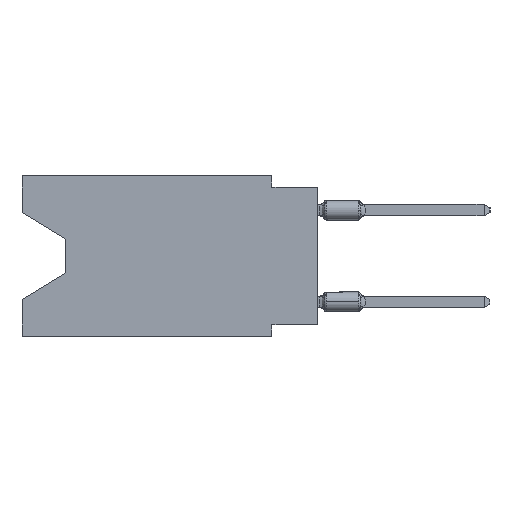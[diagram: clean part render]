
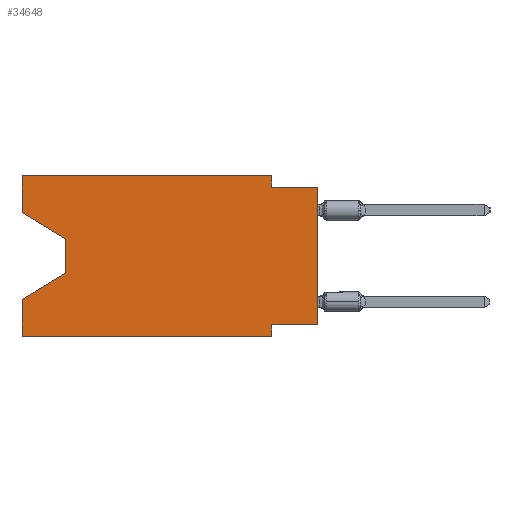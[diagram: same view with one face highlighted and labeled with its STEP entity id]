
A CAD part, left-side view. The second image highlights one B-rep face of the part: STEP entity #34648.
In plain terms, the highlighted planar face has unit normal (-1, 0, 0).
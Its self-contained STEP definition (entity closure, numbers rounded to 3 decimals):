
#612 = CARTESIAN_POINT ( 'NONE',  ( 0., 16.383, -2.038 ) ) ;
#839 = VECTOR ( 'NONE', #7871, 1000. ) ;
#1171 = EDGE_CURVE ( 'NONE', #26088, #17224, #35186, .T. ) ;
#1214 = VERTEX_POINT ( 'NONE', #32390 ) ;
#1535 = EDGE_CURVE ( 'NONE', #28753, #13794, #11944, .T. ) ;
#1687 = EDGE_CURVE ( 'NONE', #27810, #31201, #30446, .T. ) ;
#2777 = LINE ( 'NONE', #36775, #5732 ) ;
#3425 = CARTESIAN_POINT ( 'NONE',  ( 0., 16.383, 0. ) ) ;
#3776 = DIRECTION ( 'NONE',  ( 0., 0., 1. ) ) ;
#4804 = ORIENTED_EDGE ( 'NONE', *, *, #29237, .F. ) ;
#5156 = VECTOR ( 'NONE', #9319, 1000. ) ;
#5525 = EDGE_CURVE ( 'NONE', #13794, #11250, #17194, .T. ) ;
#5732 = VECTOR ( 'NONE', #28670, 1000. ) ;
#6398 = DIRECTION ( 'NONE',  ( 0., -1., 0. ) ) ;
#6976 = VECTOR ( 'NONE', #7171, 1000. ) ;
#7171 = DIRECTION ( 'NONE',  ( 0., -1., 0. ) ) ;
#7252 = ORIENTED_EDGE ( 'NONE', *, *, #5525, .F. ) ;
#7714 = CARTESIAN_POINT ( 'NONE',  ( 0., 16.383, -6.852 ) ) ;
#7871 = DIRECTION ( 'NONE',  ( 0., 0., -1. ) ) ;
#8777 = EDGE_LOOP ( 'NONE', ( #12455, #16822, #10745, #16127, #31395, #31685, #4804, #11117, #10557, #10235, #7252, #36905 ) ) ;
#9194 = PLANE ( 'NONE',  #30780 ) ;
#9319 = DIRECTION ( 'NONE',  ( 0., -1., 0. ) ) ;
#9607 = EDGE_CURVE ( 'NONE', #31598, #17224, #24558, .T. ) ;
#9770 = CARTESIAN_POINT ( 'NONE',  ( 0., 13.97, -3.505 ) ) ;
#10235 = ORIENTED_EDGE ( 'NONE', *, *, #22804, .F. ) ;
#10408 = CARTESIAN_POINT ( 'NONE',  ( 0., 16.383, -8.89 ) ) ;
#10535 = DIRECTION ( 'NONE',  ( 0., 1., 0. ) ) ;
#10557 = ORIENTED_EDGE ( 'NONE', *, *, #1171, .F. ) ;
#10745 = ORIENTED_EDGE ( 'NONE', *, *, #22064, .T. ) ;
#11117 = ORIENTED_EDGE ( 'NONE', *, *, #9607, .T. ) ;
#11250 = VERTEX_POINT ( 'NONE', #16085 ) ;
#11641 = VECTOR ( 'NONE', #25278, 1000. ) ;
#11944 = LINE ( 'NONE', #3425, #13034 ) ;
#12058 = DIRECTION ( 'NONE',  ( 1., 0., 0. ) ) ;
#12455 = ORIENTED_EDGE ( 'NONE', *, *, #27439, .T. ) ;
#12550 = EDGE_CURVE ( 'NONE', #27810, #32612, #2777, .T. ) ;
#13034 = VECTOR ( 'NONE', #3776, 1000. ) ;
#13794 = VERTEX_POINT ( 'NONE', #22152 ) ;
#14617 = CARTESIAN_POINT ( 'NONE',  ( 0., 0., -0.635 ) ) ;
#16085 = CARTESIAN_POINT ( 'NONE',  ( 0., 2.54, 0. ) ) ;
#16127 = ORIENTED_EDGE ( 'NONE', *, *, #12550, .F. ) ;
#16262 = CARTESIAN_POINT ( 'NONE',  ( 0., 0., 0. ) ) ;
#16400 = LINE ( 'NONE', #9770, #31099 ) ;
#16822 = ORIENTED_EDGE ( 'NONE', *, *, #27876, .T. ) ;
#17194 = LINE ( 'NONE', #34553, #32298 ) ;
#17224 = VERTEX_POINT ( 'NONE', #28075 ) ;
#17714 = DIRECTION ( 'NONE',  ( 0., 0., -1. ) ) ;
#17770 = CARTESIAN_POINT ( 'NONE',  ( 0., 16.383, -2.038 ) ) ;
#18477 = DIRECTION ( 'NONE',  ( 0., 0., -1. ) ) ;
#18829 = CARTESIAN_POINT ( 'NONE',  ( 0., 0., -8.255 ) ) ;
#19217 = CARTESIAN_POINT ( 'NONE',  ( 0., 2.54, -8.89 ) ) ;
#19978 = FACE_OUTER_BOUND ( 'NONE', #8777, .T. ) ;
#21249 = CARTESIAN_POINT ( 'NONE',  ( 0., 16.383, 0. ) ) ;
#22064 = EDGE_CURVE ( 'NONE', #1214, #32612, #22289, .T. ) ;
#22152 = CARTESIAN_POINT ( 'NONE',  ( 0., 16.383, 0. ) ) ;
#22289 = LINE ( 'NONE', #30831, #32125 ) ;
#22804 = EDGE_CURVE ( 'NONE', #11250, #26088, #36228, .T. ) ;
#23077 = VECTOR ( 'NONE', #10535, 1000. ) ;
#23083 = LINE ( 'NONE', #612, #34643 ) ;
#24558 = LINE ( 'NONE', #16262, #32886 ) ;
#25278 = DIRECTION ( 'NONE',  ( 0., 0., -1. ) ) ;
#26088 = VERTEX_POINT ( 'NONE', #31105 ) ;
#26640 = CARTESIAN_POINT ( 'NONE',  ( 0., 13.97, -3.505 ) ) ;
#26789 = EDGE_CURVE ( 'NONE', #32186, #31201, #37316, .T. ) ;
#27439 = EDGE_CURVE ( 'NONE', #28753, #28759, #23083, .T. ) ;
#27572 = CARTESIAN_POINT ( 'NONE',  ( 0., 2.54, 0. ) ) ;
#27810 = VERTEX_POINT ( 'NONE', #32646 ) ;
#27876 = EDGE_CURVE ( 'NONE', #28759, #1214, #16400, .T. ) ;
#28075 = CARTESIAN_POINT ( 'NONE',  ( 0., 0., -0.635 ) ) ;
#28670 = DIRECTION ( 'NONE',  ( 0., 0., 1. ) ) ;
#28753 = VERTEX_POINT ( 'NONE', #17770 ) ;
#28759 = VERTEX_POINT ( 'NONE', #26640 ) ;
#29237 = EDGE_CURVE ( 'NONE', #31598, #32186, #36026, .T. ) ;
#30446 = LINE ( 'NONE', #10408, #6976 ) ;
#30780 = AXIS2_PLACEMENT_3D ( 'NONE', #21249, #12058, #17714 ) ;
#30831 = CARTESIAN_POINT ( 'NONE',  ( 0., 13.97, -5.385 ) ) ;
#30947 = CARTESIAN_POINT ( 'NONE',  ( 0., 2.54, -8.89 ) ) ;
#31099 = VECTOR ( 'NONE', #18477, 1000. ) ;
#31105 = CARTESIAN_POINT ( 'NONE',  ( 0., 2.54, -0.635 ) ) ;
#31201 = VERTEX_POINT ( 'NONE', #19217 ) ;
#31395 = ORIENTED_EDGE ( 'NONE', *, *, #1687, .T. ) ;
#31598 = VERTEX_POINT ( 'NONE', #35405 ) ;
#31685 = ORIENTED_EDGE ( 'NONE', *, *, #26789, .F. ) ;
#32125 = VECTOR ( 'NONE', #33833, 1000. ) ;
#32186 = VERTEX_POINT ( 'NONE', #36937 ) ;
#32298 = VECTOR ( 'NONE', #6398, 1000. ) ;
#32382 = DIRECTION ( 'NONE',  ( 0., -0.855, -0.519 ) ) ;
#32390 = CARTESIAN_POINT ( 'NONE',  ( 0., 13.97, -5.385 ) ) ;
#32612 = VERTEX_POINT ( 'NONE', #7714 ) ;
#32646 = CARTESIAN_POINT ( 'NONE',  ( 0., 16.383, -8.89 ) ) ;
#32886 = VECTOR ( 'NONE', #36091, 1000. ) ;
#33833 = DIRECTION ( 'NONE',  ( 0., 0.855, -0.519 ) ) ;
#34553 = CARTESIAN_POINT ( 'NONE',  ( 0., 16.383, 0. ) ) ;
#34643 = VECTOR ( 'NONE', #32382, 1000. ) ;
#34648 = ADVANCED_FACE ( 'NONE', ( #19978 ), #9194, .F. ) ;
#35186 = LINE ( 'NONE', #14617, #5156 ) ;
#35405 = CARTESIAN_POINT ( 'NONE',  ( 0., 0., -8.255 ) ) ;
#36026 = LINE ( 'NONE', #18829, #23077 ) ;
#36091 = DIRECTION ( 'NONE',  ( 0., 0., 1. ) ) ;
#36228 = LINE ( 'NONE', #27572, #11641 ) ;
#36775 = CARTESIAN_POINT ( 'NONE',  ( 0., 16.383, 0. ) ) ;
#36905 = ORIENTED_EDGE ( 'NONE', *, *, #1535, .F. ) ;
#36937 = CARTESIAN_POINT ( 'NONE',  ( 0., 2.54, -8.255 ) ) ;
#37316 = LINE ( 'NONE', #30947, #839 ) ;
